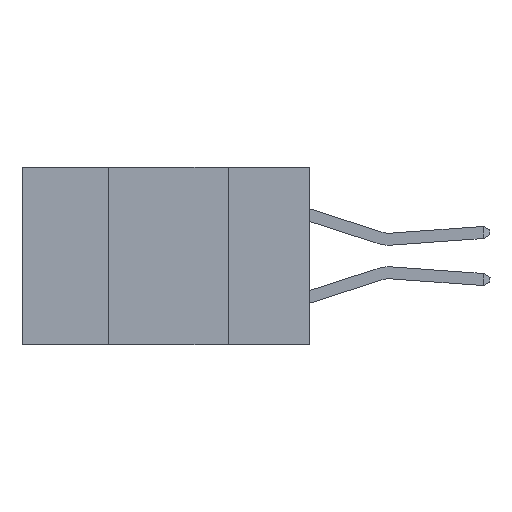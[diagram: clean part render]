
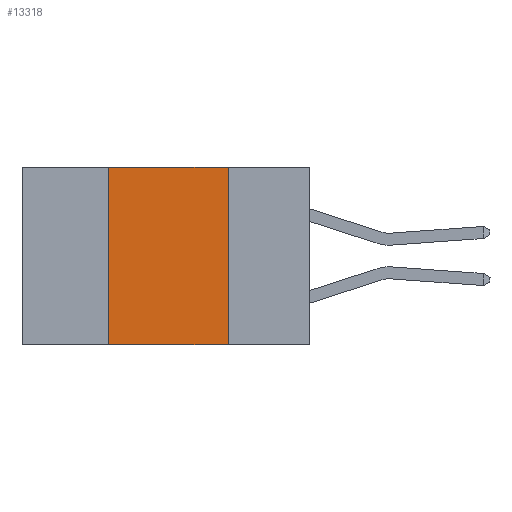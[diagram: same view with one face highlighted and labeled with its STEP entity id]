
A CAD part, left-side view. The second image highlights one B-rep face of the part: STEP entity #13318.
In plain terms, the highlighted planar face has unit normal (-1, 0, 0).
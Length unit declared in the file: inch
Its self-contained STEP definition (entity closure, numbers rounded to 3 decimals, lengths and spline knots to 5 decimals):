
#1817 = VERTEX_POINT ( 'NONE', #17225 ) ;
#2128 = CARTESIAN_POINT ( 'NONE',  ( 0., 0.6, -0.37 ) ) ;
#2742 = AXIS2_PLACEMENT_3D ( 'NONE', #9997, #5880, #20371 ) ;
#3758 = PLANE ( 'NONE',  #2742 ) ;
#4819 = CARTESIAN_POINT ( 'NONE',  ( 0., 0.17, -0.37 ) ) ;
#5066 = LINE ( 'NONE', #4819, #25691 ) ;
#5273 = ORIENTED_EDGE ( 'NONE', *, *, #23020, .F. ) ;
#5880 = DIRECTION ( 'NONE',  ( 1., 0., 0. ) ) ;
#6543 = VERTEX_POINT ( 'NONE', #16270 ) ;
#7698 = VECTOR ( 'NONE', #11097, 39.37008 ) ;
#7903 = CARTESIAN_POINT ( 'NONE',  ( 0., 0.42, -0.37 ) ) ;
#7947 = VECTOR ( 'NONE', #12087, 39.37008 ) ;
#8034 = VECTOR ( 'NONE', #26384, 39.37008 ) ;
#9997 = CARTESIAN_POINT ( 'NONE',  ( 0., 0.6, 0. ) ) ;
#10111 = EDGE_CURVE ( 'NONE', #1817, #15775, #24439, .T. ) ;
#10397 = VERTEX_POINT ( 'NONE', #19536 ) ;
#10841 = EDGE_LOOP ( 'NONE', ( #13728, #5273, #26550, #14842 ) ) ;
#11097 = DIRECTION ( 'NONE',  ( 0., -1., 0. ) ) ;
#11429 = FACE_OUTER_BOUND ( 'NONE', #10841, .T. ) ;
#12087 = DIRECTION ( 'NONE',  ( 0., 0., 1. ) ) ;
#12569 = LINE ( 'NONE', #23388, #7698 ) ;
#13318 = ADVANCED_FACE ( 'NONE', ( #11429 ), #3758, .F. ) ;
#13728 = ORIENTED_EDGE ( 'NONE', *, *, #16196, .F. ) ;
#14842 = ORIENTED_EDGE ( 'NONE', *, *, #10111, .T. ) ;
#15775 = VERTEX_POINT ( 'NONE', #21705 ) ;
#16196 = EDGE_CURVE ( 'NONE', #10397, #15775, #5066, .T. ) ;
#16270 = CARTESIAN_POINT ( 'NONE',  ( 0., 0.42, 0. ) ) ;
#17225 = CARTESIAN_POINT ( 'NONE',  ( 0., 0.42, -0.37 ) ) ;
#19536 = CARTESIAN_POINT ( 'NONE',  ( 0., 0.17, 0. ) ) ;
#20371 = DIRECTION ( 'NONE',  ( 0., 0., -1. ) ) ;
#21705 = CARTESIAN_POINT ( 'NONE',  ( 0., 0.17, -0.37 ) ) ;
#23020 = EDGE_CURVE ( 'NONE', #6543, #10397, #12569, .T. ) ;
#23388 = CARTESIAN_POINT ( 'NONE',  ( 0., 0.6, 0. ) ) ;
#24348 = LINE ( 'NONE', #7903, #7947 ) ;
#24439 = LINE ( 'NONE', #2128, #8034 ) ;
#25234 = EDGE_CURVE ( 'NONE', #1817, #6543, #24348, .T. ) ;
#25474 = DIRECTION ( 'NONE',  ( 0., 0., -1. ) ) ;
#25691 = VECTOR ( 'NONE', #25474, 39.37008 ) ;
#26384 = DIRECTION ( 'NONE',  ( 0., -1., 0. ) ) ;
#26550 = ORIENTED_EDGE ( 'NONE', *, *, #25234, .F. ) ;
